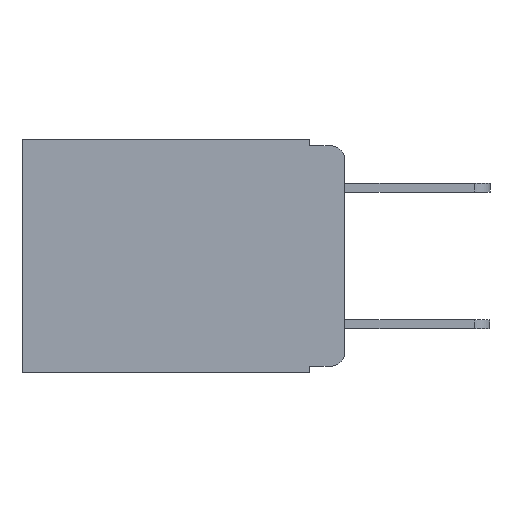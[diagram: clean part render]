
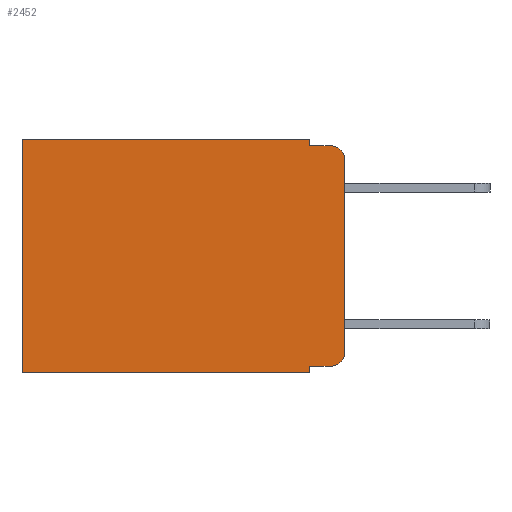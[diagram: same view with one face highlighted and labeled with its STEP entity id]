
A CAD part, left-side view. The second image highlights one B-rep face of the part: STEP entity #2452.
In plain terms, the highlighted planar face has unit normal (-1, 0, 0).
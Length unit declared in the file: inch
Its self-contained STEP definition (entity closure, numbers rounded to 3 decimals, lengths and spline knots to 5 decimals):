
#67 = VERTEX_POINT ( 'NONE', #3910 ) ;
#283 = LINE ( 'NONE', #6865, #3784 ) ;
#745 = AXIS2_PLACEMENT_3D ( 'NONE', #5974, #5301, #5270 ) ;
#747 = AXIS2_PLACEMENT_3D ( 'NONE', #7252, #11279, #1184 ) ;
#754 = DIRECTION ( 'NONE',  ( 0., -1., 0. ) ) ;
#907 = VERTEX_POINT ( 'NONE', #10178 ) ;
#1090 = DIRECTION ( 'NONE',  ( 0., -1., 0. ) ) ;
#1184 = DIRECTION ( 'NONE',  ( 0., 0., -1. ) ) ;
#1625 = ORIENTED_EDGE ( 'NONE', *, *, #4620, .F. ) ;
#1638 = VECTOR ( 'NONE', #1090, 39.37008 ) ;
#2289 = VECTOR ( 'NONE', #754, 39.37008 ) ;
#2295 = ORIENTED_EDGE ( 'NONE', *, *, #4587, .F. ) ;
#2296 = CARTESIAN_POINT ( 'NONE',  ( 0.298, 0.051, 0. ) ) ;
#2302 = VERTEX_POINT ( 'NONE', #9937 ) ;
#2452 = ADVANCED_FACE ( 'NONE', ( #10034 ), #3839, .F. ) ;
#2611 = ORIENTED_EDGE ( 'NONE', *, *, #4604, .T. ) ;
#2645 = VECTOR ( 'NONE', #7077, 39.37008 ) ;
#3099 = VERTEX_POINT ( 'NONE', #10059 ) ;
#3419 = CARTESIAN_POINT ( 'NONE',  ( 0.298, 0.473, -0.343 ) ) ;
#3648 = CARTESIAN_POINT ( 'NONE',  ( 0.298, 0., 0. ) ) ;
#3685 = ORIENTED_EDGE ( 'NONE', *, *, #4651, .F. ) ;
#3784 = VECTOR ( 'NONE', #10354, 39.37008 ) ;
#3839 = PLANE ( 'NONE',  #3993 ) ;
#3910 = CARTESIAN_POINT ( 'NONE',  ( 0.298, 0.02, -0.333 ) ) ;
#3964 = DIRECTION ( 'NONE',  ( 0., 0., -1. ) ) ;
#3973 = CARTESIAN_POINT ( 'NONE',  ( 0.298, 0.051, -0.01 ) ) ;
#3983 = EDGE_CURVE ( 'NONE', #6428, #3099, #9032, .T. ) ;
#3993 = AXIS2_PLACEMENT_3D ( 'NONE', #8309, #8278, #5746 ) ;
#4009 = VERTEX_POINT ( 'NONE', #9212 ) ;
#4220 = DIRECTION ( 'NONE',  ( 0., 1., 0. ) ) ;
#4281 = VECTOR ( 'NONE', #4220, 39.37008 ) ;
#4344 = EDGE_CURVE ( 'NONE', #4009, #9051, #283, .T. ) ;
#4416 = CIRCLE ( 'NONE', #745, 0.02 ) ;
#4587 = EDGE_CURVE ( 'NONE', #7784, #8793, #9815, .T. ) ;
#4604 = EDGE_CURVE ( 'NONE', #7784, #10562, #8045, .T. ) ;
#4620 = EDGE_CURVE ( 'NONE', #907, #10562, #11313, .T. ) ;
#4638 = EDGE_CURVE ( 'NONE', #6428, #907, #9361, .T. ) ;
#4650 = EDGE_CURVE ( 'NONE', #3099, #9051, #7494, .T. ) ;
#4651 = EDGE_CURVE ( 'NONE', #2302, #4009, #4704, .T. ) ;
#4672 = EDGE_CURVE ( 'NONE', #2302, #67, #9131, .T. ) ;
#4687 = EDGE_CURVE ( 'NONE', #67, #8793, #4416, .T. ) ;
#4704 = LINE ( 'NONE', #2296, #10910 ) ;
#4707 = CARTESIAN_POINT ( 'NONE',  ( 0.298, 0., 0. ) ) ;
#4870 = ORIENTED_EDGE ( 'NONE', *, *, #4672, .T. ) ;
#4989 = VECTOR ( 'NONE', #3964, 39.37008 ) ;
#4990 = EDGE_LOOP ( 'NONE', ( #2295, #2611, #1625, #8948, #9953, #5211, #5105, #3685, #4870, #10651 ) ) ;
#5105 = ORIENTED_EDGE ( 'NONE', *, *, #4344, .F. ) ;
#5211 = ORIENTED_EDGE ( 'NONE', *, *, #4650, .T. ) ;
#5270 = DIRECTION ( 'NONE',  ( 0., 0., -1. ) ) ;
#5301 = DIRECTION ( 'NONE',  ( -1., 0., 0. ) ) ;
#5746 = DIRECTION ( 'NONE',  ( 0., 0., -1. ) ) ;
#5974 = CARTESIAN_POINT ( 'NONE',  ( 0.298, 0.02, -0.313 ) ) ;
#6128 = CARTESIAN_POINT ( 'NONE',  ( 0.298, 0., -0.313 ) ) ;
#6428 = VERTEX_POINT ( 'NONE', #11170 ) ;
#6865 = CARTESIAN_POINT ( 'NONE',  ( 0.298, 0., -0.343 ) ) ;
#7077 = DIRECTION ( 'NONE',  ( 0., 0., -1. ) ) ;
#7212 = VECTOR ( 'NONE', #11217, 39.37008 ) ;
#7252 = CARTESIAN_POINT ( 'NONE',  ( 0.298, 0.02, -0.03 ) ) ;
#7494 = LINE ( 'NONE', #8747, #4989 ) ;
#7784 = VERTEX_POINT ( 'NONE', #11452 ) ;
#8045 = CIRCLE ( 'NONE', #747, 0.02 ) ;
#8278 = DIRECTION ( 'NONE',  ( 1., 0., 0. ) ) ;
#8309 = CARTESIAN_POINT ( 'NONE',  ( 0.298, 0., 0. ) ) ;
#8747 = CARTESIAN_POINT ( 'NONE',  ( 0.298, 0.473, 0. ) ) ;
#8793 = VERTEX_POINT ( 'NONE', #6128 ) ;
#8935 = CARTESIAN_POINT ( 'NONE',  ( 0.298, 0.051, 0. ) ) ;
#8948 = ORIENTED_EDGE ( 'NONE', *, *, #4638, .F. ) ;
#9032 = LINE ( 'NONE', #4707, #4281 ) ;
#9051 = VERTEX_POINT ( 'NONE', #3419 ) ;
#9131 = LINE ( 'NONE', #10166, #1638 ) ;
#9163 = CARTESIAN_POINT ( 'NONE',  ( 0.298, 0.02, -0.01 ) ) ;
#9212 = CARTESIAN_POINT ( 'NONE',  ( 0.298, 0.051, -0.343 ) ) ;
#9361 = LINE ( 'NONE', #8935, #7212 ) ;
#9815 = LINE ( 'NONE', #3648, #2645 ) ;
#9937 = CARTESIAN_POINT ( 'NONE',  ( 0.298, 0.051, -0.333 ) ) ;
#9953 = ORIENTED_EDGE ( 'NONE', *, *, #3983, .T. ) ;
#10034 = FACE_OUTER_BOUND ( 'NONE', #4990, .T. ) ;
#10059 = CARTESIAN_POINT ( 'NONE',  ( 0.298, 0.473, 0. ) ) ;
#10166 = CARTESIAN_POINT ( 'NONE',  ( 0.298, 0.051, -0.333 ) ) ;
#10178 = CARTESIAN_POINT ( 'NONE',  ( 0.298, 0.051, -0.01 ) ) ;
#10354 = DIRECTION ( 'NONE',  ( 0., 1., 0. ) ) ;
#10562 = VERTEX_POINT ( 'NONE', #9163 ) ;
#10651 = ORIENTED_EDGE ( 'NONE', *, *, #4687, .T. ) ;
#10910 = VECTOR ( 'NONE', #11185, 39.37008 ) ;
#11170 = CARTESIAN_POINT ( 'NONE',  ( 0.298, 0.051, 0. ) ) ;
#11185 = DIRECTION ( 'NONE',  ( 0., 0., -1. ) ) ;
#11217 = DIRECTION ( 'NONE',  ( 0., 0., -1. ) ) ;
#11279 = DIRECTION ( 'NONE',  ( -1., 0., 0. ) ) ;
#11313 = LINE ( 'NONE', #3973, #2289 ) ;
#11452 = CARTESIAN_POINT ( 'NONE',  ( 0.298, 0., -0.03 ) ) ;
